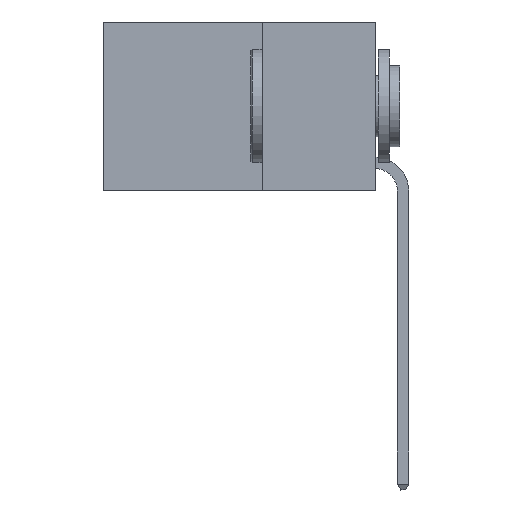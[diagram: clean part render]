
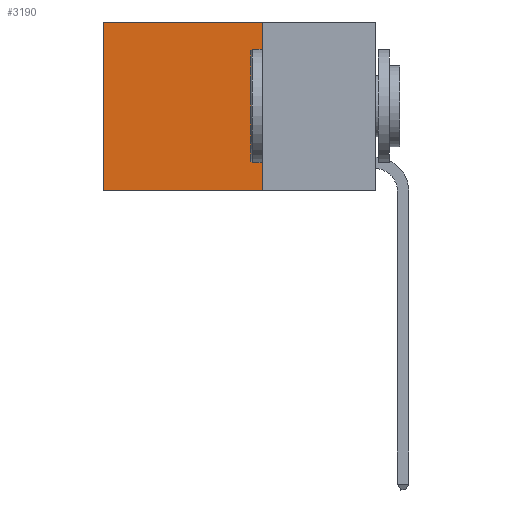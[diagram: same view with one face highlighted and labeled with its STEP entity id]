
A CAD part, left-side view. The second image highlights one B-rep face of the part: STEP entity #3190.
In plain terms, the highlighted planar face has unit normal (-1, 0, 0).
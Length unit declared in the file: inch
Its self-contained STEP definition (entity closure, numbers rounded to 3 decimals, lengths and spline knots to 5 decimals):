
#595 = VECTOR ( 'NONE', #4101, 39.37008 ) ;
#942 = CARTESIAN_POINT ( 'NONE',  ( 0.2625, 0.25, 0. ) ) ;
#1079 = ORIENTED_EDGE ( 'NONE', *, *, #10580, .F. ) ;
#1357 = CARTESIAN_POINT ( 'NONE',  ( 0.2625, 0.25, 0. ) ) ;
#1365 = DIRECTION ( 'NONE',  ( 0., 1., 0. ) ) ;
#2639 = EDGE_CURVE ( 'NONE', #12645, #10844, #5775, .T. ) ;
#2966 = CARTESIAN_POINT ( 'NONE',  ( 0.2625, 0.25, 0. ) ) ;
#3181 = EDGE_CURVE ( 'NONE', #10844, #6485, #12755, .T. ) ;
#3190 = ADVANCED_FACE ( 'NONE', ( #4959 ), #8339, .F. ) ;
#3260 = VECTOR ( 'NONE', #10512, 39.37008 ) ;
#3531 = CARTESIAN_POINT ( 'NONE',  ( 0.2625, 0.6, 0. ) ) ;
#4101 = DIRECTION ( 'NONE',  ( 0., 0., -1. ) ) ;
#4195 = EDGE_LOOP ( 'NONE', ( #4597, #1079, #10981, #5264 ) ) ;
#4597 = ORIENTED_EDGE ( 'NONE', *, *, #3181, .T. ) ;
#4959 = FACE_OUTER_BOUND ( 'NONE', #4195, .T. ) ;
#5264 = ORIENTED_EDGE ( 'NONE', *, *, #2639, .T. ) ;
#5330 = VECTOR ( 'NONE', #7936, 39.37008 ) ;
#5775 = LINE ( 'NONE', #1357, #5330 ) ;
#6485 = VERTEX_POINT ( 'NONE', #6571 ) ;
#6571 = CARTESIAN_POINT ( 'NONE',  ( 0.2625, 0.6, -0.37 ) ) ;
#6800 = LINE ( 'NONE', #11144, #11870 ) ;
#7220 = EDGE_CURVE ( 'NONE', #12645, #14074, #13944, .T. ) ;
#7936 = DIRECTION ( 'NONE',  ( 0., 1., 0. ) ) ;
#8196 = DIRECTION ( 'NONE',  ( 1., 0., 0. ) ) ;
#8339 = PLANE ( 'NONE',  #14061 ) ;
#8519 = CARTESIAN_POINT ( 'NONE',  ( 0.2625, 0.25, 0. ) ) ;
#10151 = CARTESIAN_POINT ( 'NONE',  ( 0.2625, 0.25, -0.37 ) ) ;
#10512 = DIRECTION ( 'NONE',  ( 0., 0., -1. ) ) ;
#10580 = EDGE_CURVE ( 'NONE', #14074, #6485, #6800, .T. ) ;
#10844 = VERTEX_POINT ( 'NONE', #3531 ) ;
#10981 = ORIENTED_EDGE ( 'NONE', *, *, #7220, .F. ) ;
#11144 = CARTESIAN_POINT ( 'NONE',  ( 0.2625, 0.25, -0.37 ) ) ;
#11660 = DIRECTION ( 'NONE',  ( 0., 0., -1. ) ) ;
#11870 = VECTOR ( 'NONE', #1365, 39.37008 ) ;
#12616 = CARTESIAN_POINT ( 'NONE',  ( 0.2625, 0.6, 0. ) ) ;
#12645 = VERTEX_POINT ( 'NONE', #8519 ) ;
#12755 = LINE ( 'NONE', #12616, #595 ) ;
#13944 = LINE ( 'NONE', #942, #3260 ) ;
#14061 = AXIS2_PLACEMENT_3D ( 'NONE', #2966, #8196, #11660 ) ;
#14074 = VERTEX_POINT ( 'NONE', #10151 ) ;
